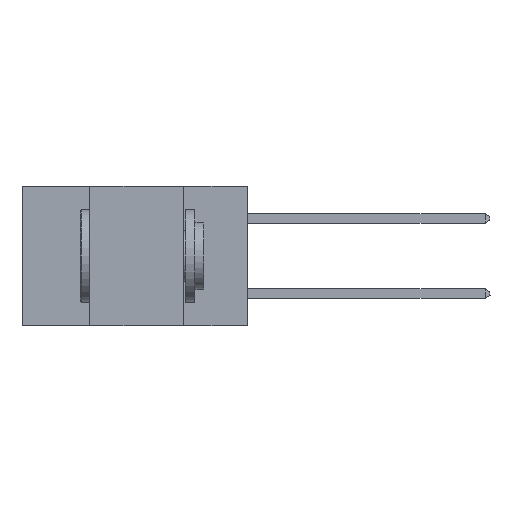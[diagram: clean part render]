
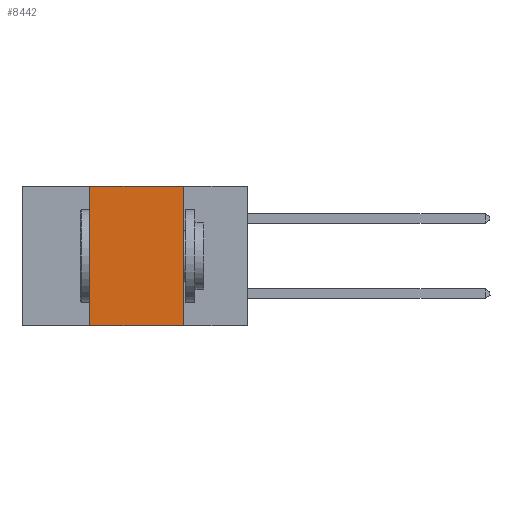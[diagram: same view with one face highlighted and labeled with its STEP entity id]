
A CAD part, left-side view. The second image highlights one B-rep face of the part: STEP entity #8442.
In plain terms, the highlighted planar face has unit normal (-1, 0, 0).
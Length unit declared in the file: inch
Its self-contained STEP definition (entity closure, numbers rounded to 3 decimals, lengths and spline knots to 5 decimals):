
#72 = VERTEX_POINT ( 'NONE', #23630 ) ;
#400 = EDGE_CURVE ( 'NONE', #72, #18508, #26726, .T. ) ;
#482 = VECTOR ( 'NONE', #9240, 39.37008 ) ;
#483 = CARTESIAN_POINT ( 'NONE',  ( 0., 0.17, 0. ) ) ;
#578 = VECTOR ( 'NONE', #14769, 39.37008 ) ;
#630 = DIRECTION ( 'NONE',  ( 0., -1., 0. ) ) ;
#967 = CARTESIAN_POINT ( 'NONE',  ( 0., 0.42, -0.37 ) ) ;
#1687 = CARTESIAN_POINT ( 'NONE',  ( 0., 0.42, 0. ) ) ;
#4816 = ORIENTED_EDGE ( 'NONE', *, *, #9631, .T. ) ;
#5279 = PLANE ( 'NONE',  #18987 ) ;
#7966 = VERTEX_POINT ( 'NONE', #25357 ) ;
#8442 = ADVANCED_FACE ( 'NONE', ( #19441 ), #5279, .F. ) ;
#9240 = DIRECTION ( 'NONE',  ( 0., 0., -1. ) ) ;
#9631 = EDGE_CURVE ( 'NONE', #10768, #7966, #12090, .T. ) ;
#9771 = ORIENTED_EDGE ( 'NONE', *, *, #28066, .F. ) ;
#10018 = LINE ( 'NONE', #1687, #21498 ) ;
#10768 = VERTEX_POINT ( 'NONE', #967 ) ;
#11652 = CARTESIAN_POINT ( 'NONE',  ( 0., 0.6, 0. ) ) ;
#12090 = LINE ( 'NONE', #19243, #578 ) ;
#12326 = LINE ( 'NONE', #25188, #482 ) ;
#12729 = EDGE_LOOP ( 'NONE', ( #9771, #26878, #16390, #4816 ) ) ;
#14148 = CARTESIAN_POINT ( 'NONE',  ( 0., 0.6, 0. ) ) ;
#14769 = DIRECTION ( 'NONE',  ( 0., -1., 0. ) ) ;
#14992 = EDGE_CURVE ( 'NONE', #10768, #72, #10018, .T. ) ;
#16390 = ORIENTED_EDGE ( 'NONE', *, *, #14992, .F. ) ;
#18508 = VERTEX_POINT ( 'NONE', #483 ) ;
#18987 = AXIS2_PLACEMENT_3D ( 'NONE', #14148, #20684, #25335 ) ;
#19243 = CARTESIAN_POINT ( 'NONE',  ( 0., 0.6, -0.37 ) ) ;
#19441 = FACE_OUTER_BOUND ( 'NONE', #12729, .T. ) ;
#20684 = DIRECTION ( 'NONE',  ( 1., 0., 0. ) ) ;
#20807 = VECTOR ( 'NONE', #630, 39.37008 ) ;
#21498 = VECTOR ( 'NONE', #25928, 39.37008 ) ;
#23630 = CARTESIAN_POINT ( 'NONE',  ( 0., 0.42, 0. ) ) ;
#25188 = CARTESIAN_POINT ( 'NONE',  ( 0., 0.17, 0. ) ) ;
#25335 = DIRECTION ( 'NONE',  ( 0., 0., -1. ) ) ;
#25357 = CARTESIAN_POINT ( 'NONE',  ( 0., 0.17, -0.37 ) ) ;
#25928 = DIRECTION ( 'NONE',  ( 0., 0., 1. ) ) ;
#26726 = LINE ( 'NONE', #11652, #20807 ) ;
#26878 = ORIENTED_EDGE ( 'NONE', *, *, #400, .F. ) ;
#28066 = EDGE_CURVE ( 'NONE', #18508, #7966, #12326, .T. ) ;
